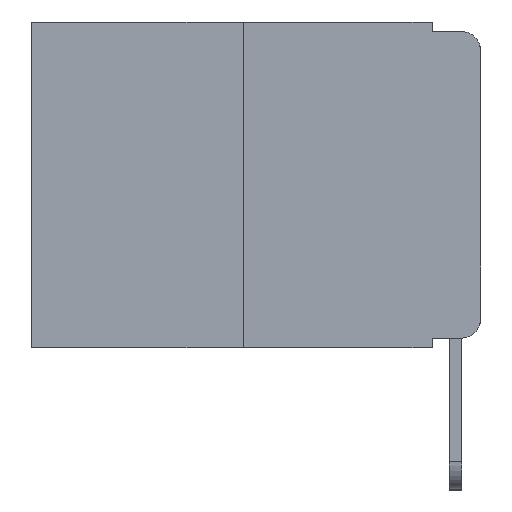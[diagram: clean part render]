
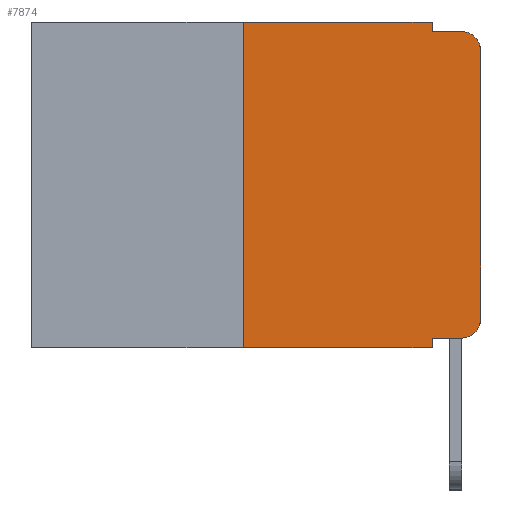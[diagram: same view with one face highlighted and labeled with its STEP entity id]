
A CAD part, left-side view. The second image highlights one B-rep face of the part: STEP entity #7874.
In plain terms, the highlighted planar face has unit normal (-1, 0, 0).
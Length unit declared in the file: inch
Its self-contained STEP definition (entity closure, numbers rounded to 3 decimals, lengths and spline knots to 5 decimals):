
#391 = ORIENTED_EDGE ( 'NONE', *, *, #12639, .F. ) ;
#586 = EDGE_CURVE ( 'NONE', #6200, #8298, #702, .T. ) ;
#694 = LINE ( 'NONE', #8469, #3132 ) ;
#702 = LINE ( 'NONE', #768, #8153 ) ;
#768 = CARTESIAN_POINT ( 'NONE',  ( 0., 0.473, -0.343 ) ) ;
#803 = DIRECTION ( 'NONE',  ( -1., 0., 0. ) ) ;
#805 = CARTESIAN_POINT ( 'NONE',  ( 0., 0.051, -0.333 ) ) ;
#825 = VERTEX_POINT ( 'NONE', #13710 ) ;
#830 = AXIS2_PLACEMENT_3D ( 'NONE', #3190, #13360, #12126 ) ;
#979 = LINE ( 'NONE', #4957, #8693 ) ;
#1062 = CIRCLE ( 'NONE', #830, 0.02 ) ;
#1100 = VECTOR ( 'NONE', #5921, 39.37008 ) ;
#1304 = CIRCLE ( 'NONE', #10525, 0.02 ) ;
#1355 = ORIENTED_EDGE ( 'NONE', *, *, #2740, .T. ) ;
#1400 = CARTESIAN_POINT ( 'NONE',  ( 0., 0.25, 0. ) ) ;
#1935 = DIRECTION ( 'NONE',  ( 0., 0., -1. ) ) ;
#2060 = DIRECTION ( 'NONE',  ( 0., -1., 0. ) ) ;
#2124 = CARTESIAN_POINT ( 'NONE',  ( 0., 0.051, -0.343 ) ) ;
#2210 = CARTESIAN_POINT ( 'NONE',  ( 0., 0.051, -0.333 ) ) ;
#2521 = ORIENTED_EDGE ( 'NONE', *, *, #3088, .F. ) ;
#2525 = ORIENTED_EDGE ( 'NONE', *, *, #3840, .F. ) ;
#2526 = CARTESIAN_POINT ( 'NONE',  ( 0., 0.02, -0.01 ) ) ;
#2654 = DIRECTION ( 'NONE',  ( 0., 0., -1. ) ) ;
#2740 = EDGE_CURVE ( 'NONE', #11367, #4956, #1304, .T. ) ;
#2869 = EDGE_CURVE ( 'NONE', #825, #10224, #1062, .T. ) ;
#3088 = EDGE_CURVE ( 'NONE', #3978, #8298, #5110, .T. ) ;
#3132 = VECTOR ( 'NONE', #7395, 39.37008 ) ;
#3190 = CARTESIAN_POINT ( 'NONE',  ( 0., 0.02, -0.313 ) ) ;
#3268 = EDGE_CURVE ( 'NONE', #3978, #825, #8995, .T. ) ;
#3521 = ORIENTED_EDGE ( 'NONE', *, *, #2869, .T. ) ;
#3528 = FACE_OUTER_BOUND ( 'NONE', #11044, .T. ) ;
#3813 = VERTEX_POINT ( 'NONE', #1400 ) ;
#3840 = EDGE_CURVE ( 'NONE', #8210, #4956, #7093, .T. ) ;
#3913 = CARTESIAN_POINT ( 'NONE',  ( 0., 0.02, -0.03 ) ) ;
#3978 = VERTEX_POINT ( 'NONE', #805 ) ;
#4297 = DIRECTION ( 'NONE',  ( 0., 0., -1. ) ) ;
#4598 = CARTESIAN_POINT ( 'NONE',  ( 0., 0., -0.313 ) ) ;
#4634 = ORIENTED_EDGE ( 'NONE', *, *, #5002, .F. ) ;
#4956 = VERTEX_POINT ( 'NONE', #2526 ) ;
#4957 = CARTESIAN_POINT ( 'NONE',  ( 0., 0., 0. ) ) ;
#4985 = DIRECTION ( 'NONE',  ( 0., -1., 0. ) ) ;
#5002 = EDGE_CURVE ( 'NONE', #3813, #7119, #7131, .T. ) ;
#5110 = LINE ( 'NONE', #8365, #12820 ) ;
#5766 = LINE ( 'NONE', #5913, #13580 ) ;
#5913 = CARTESIAN_POINT ( 'NONE',  ( 0., 0.051, 0. ) ) ;
#5921 = DIRECTION ( 'NONE',  ( 0., -1., 0. ) ) ;
#6200 = VERTEX_POINT ( 'NONE', #8869 ) ;
#6776 = DIRECTION ( 'NONE',  ( 1., 0., 0. ) ) ;
#6885 = EDGE_CURVE ( 'NONE', #6200, #3813, #694, .T. ) ;
#7093 = LINE ( 'NONE', #9323, #10113 ) ;
#7119 = VERTEX_POINT ( 'NONE', #12438 ) ;
#7131 = LINE ( 'NONE', #8005, #1100 ) ;
#7376 = ORIENTED_EDGE ( 'NONE', *, *, #3268, .T. ) ;
#7395 = DIRECTION ( 'NONE',  ( 0., 0., 1. ) ) ;
#7760 = DIRECTION ( 'NONE',  ( 0., -1., 0. ) ) ;
#7874 = ADVANCED_FACE ( 'NONE', ( #3528 ), #13325, .F. ) ;
#8005 = CARTESIAN_POINT ( 'NONE',  ( 0., 0.473, 0. ) ) ;
#8153 = VECTOR ( 'NONE', #2060, 39.37008 ) ;
#8210 = VERTEX_POINT ( 'NONE', #10933 ) ;
#8298 = VERTEX_POINT ( 'NONE', #2124 ) ;
#8365 = CARTESIAN_POINT ( 'NONE',  ( 0., 0.051, 0. ) ) ;
#8469 = CARTESIAN_POINT ( 'NONE',  ( 0., 0.25, 0. ) ) ;
#8654 = EDGE_CURVE ( 'NONE', #10224, #11367, #979, .T. ) ;
#8693 = VECTOR ( 'NONE', #13078, 39.37008 ) ;
#8869 = CARTESIAN_POINT ( 'NONE',  ( 0., 0.25, -0.343 ) ) ;
#8995 = LINE ( 'NONE', #2210, #11445 ) ;
#9167 = ORIENTED_EDGE ( 'NONE', *, *, #8654, .T. ) ;
#9323 = CARTESIAN_POINT ( 'NONE',  ( 0., 0.051, -0.01 ) ) ;
#9615 = ORIENTED_EDGE ( 'NONE', *, *, #6885, .F. ) ;
#9806 = CARTESIAN_POINT ( 'NONE',  ( 0., 0., -0.03 ) ) ;
#10113 = VECTOR ( 'NONE', #4985, 39.37008 ) ;
#10224 = VERTEX_POINT ( 'NONE', #4598 ) ;
#10525 = AXIS2_PLACEMENT_3D ( 'NONE', #3913, #803, #11903 ) ;
#10577 = ORIENTED_EDGE ( 'NONE', *, *, #586, .T. ) ;
#10898 = AXIS2_PLACEMENT_3D ( 'NONE', #12167, #6776, #1935 ) ;
#10933 = CARTESIAN_POINT ( 'NONE',  ( 0., 0.051, -0.01 ) ) ;
#11044 = EDGE_LOOP ( 'NONE', ( #9167, #1355, #2525, #391, #4634, #9615, #10577, #2521, #7376, #3521 ) ) ;
#11367 = VERTEX_POINT ( 'NONE', #9806 ) ;
#11445 = VECTOR ( 'NONE', #7760, 39.37008 ) ;
#11903 = DIRECTION ( 'NONE',  ( 0., 0., -1. ) ) ;
#12126 = DIRECTION ( 'NONE',  ( 0., 0., -1. ) ) ;
#12167 = CARTESIAN_POINT ( 'NONE',  ( 0., 0.473, 0. ) ) ;
#12438 = CARTESIAN_POINT ( 'NONE',  ( 0., 0.051, 0. ) ) ;
#12639 = EDGE_CURVE ( 'NONE', #7119, #8210, #5766, .T. ) ;
#12820 = VECTOR ( 'NONE', #4297, 39.37008 ) ;
#13078 = DIRECTION ( 'NONE',  ( 0., 0., 1. ) ) ;
#13325 = PLANE ( 'NONE',  #10898 ) ;
#13360 = DIRECTION ( 'NONE',  ( -1., 0., 0. ) ) ;
#13580 = VECTOR ( 'NONE', #2654, 39.37008 ) ;
#13710 = CARTESIAN_POINT ( 'NONE',  ( 0., 0.02, -0.333 ) ) ;
